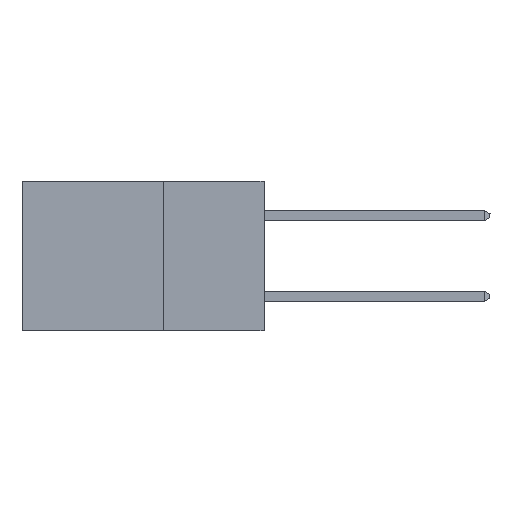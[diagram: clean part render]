
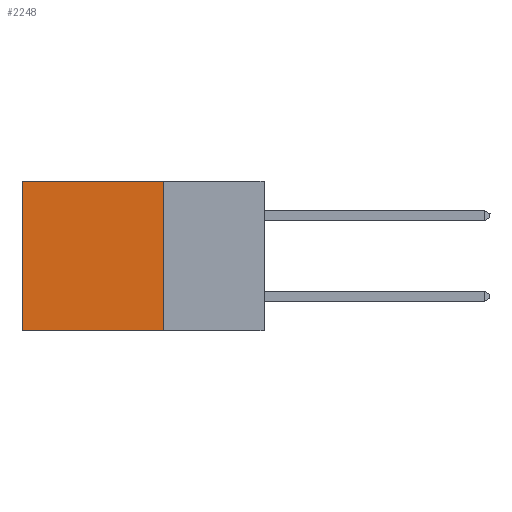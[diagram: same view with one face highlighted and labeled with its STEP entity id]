
A CAD part, left-side view. The second image highlights one B-rep face of the part: STEP entity #2248.
In plain terms, the highlighted planar face has unit normal (-1, 0, 0).
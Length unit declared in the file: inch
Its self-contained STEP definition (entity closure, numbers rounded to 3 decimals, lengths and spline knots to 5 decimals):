
#247 = ORIENTED_EDGE ( 'NONE', *, *, #20662, .T. ) ;
#549 = CARTESIAN_POINT ( 'NONE',  ( 0.298, 0.6, 0. ) ) ;
#851 = VECTOR ( 'NONE', #26185, 39.37008 ) ;
#967 = CARTESIAN_POINT ( 'NONE',  ( 0.298, 0.25, -0.37 ) ) ;
#1176 = DIRECTION ( 'NONE',  ( 1., 0., 0. ) ) ;
#1591 = DIRECTION ( 'NONE',  ( 0., 1., 0. ) ) ;
#1807 = AXIS2_PLACEMENT_3D ( 'NONE', #21509, #1176, #25706 ) ;
#2248 = ADVANCED_FACE ( 'NONE', ( #9188 ), #25797, .F. ) ;
#3129 = CARTESIAN_POINT ( 'NONE',  ( 0.298, 0.25, 0. ) ) ;
#4835 = LINE ( 'NONE', #3129, #10101 ) ;
#5157 = VERTEX_POINT ( 'NONE', #26018 ) ;
#5836 = VECTOR ( 'NONE', #1591, 39.37008 ) ;
#6272 = LINE ( 'NONE', #19733, #19415 ) ;
#9178 = ORIENTED_EDGE ( 'NONE', *, *, #21158, .F. ) ;
#9188 = FACE_OUTER_BOUND ( 'NONE', #12594, .T. ) ;
#10101 = VECTOR ( 'NONE', #21194, 39.37008 ) ;
#10630 = CARTESIAN_POINT ( 'NONE',  ( 0.298, 0.6, -0.37 ) ) ;
#10810 = EDGE_CURVE ( 'NONE', #5157, #16552, #29239, .T. ) ;
#12594 = EDGE_LOOP ( 'NONE', ( #247, #17865, #9178, #18490 ) ) ;
#12768 = CARTESIAN_POINT ( 'NONE',  ( 0.298, 0.25, -0.37 ) ) ;
#14015 = LINE ( 'NONE', #967, #851 ) ;
#16552 = VERTEX_POINT ( 'NONE', #549 ) ;
#17506 = VERTEX_POINT ( 'NONE', #10630 ) ;
#17865 = ORIENTED_EDGE ( 'NONE', *, *, #28576, .F. ) ;
#18490 = ORIENTED_EDGE ( 'NONE', *, *, #10810, .T. ) ;
#19415 = VECTOR ( 'NONE', #26403, 39.37008 ) ;
#19733 = CARTESIAN_POINT ( 'NONE',  ( 0.298, 0.6, 0. ) ) ;
#20662 = EDGE_CURVE ( 'NONE', #16552, #17506, #6272, .T. ) ;
#21158 = EDGE_CURVE ( 'NONE', #5157, #29241, #4835, .T. ) ;
#21194 = DIRECTION ( 'NONE',  ( 0., 0., -1. ) ) ;
#21509 = CARTESIAN_POINT ( 'NONE',  ( 0.298, 0.25, 0. ) ) ;
#22214 = CARTESIAN_POINT ( 'NONE',  ( 0.298, 0.25, 0. ) ) ;
#25706 = DIRECTION ( 'NONE',  ( 0., 0., -1. ) ) ;
#25797 = PLANE ( 'NONE',  #1807 ) ;
#26018 = CARTESIAN_POINT ( 'NONE',  ( 0.298, 0.25, 0. ) ) ;
#26185 = DIRECTION ( 'NONE',  ( 0., 1., 0. ) ) ;
#26403 = DIRECTION ( 'NONE',  ( 0., 0., -1. ) ) ;
#28576 = EDGE_CURVE ( 'NONE', #29241, #17506, #14015, .T. ) ;
#29239 = LINE ( 'NONE', #22214, #5836 ) ;
#29241 = VERTEX_POINT ( 'NONE', #12768 ) ;
